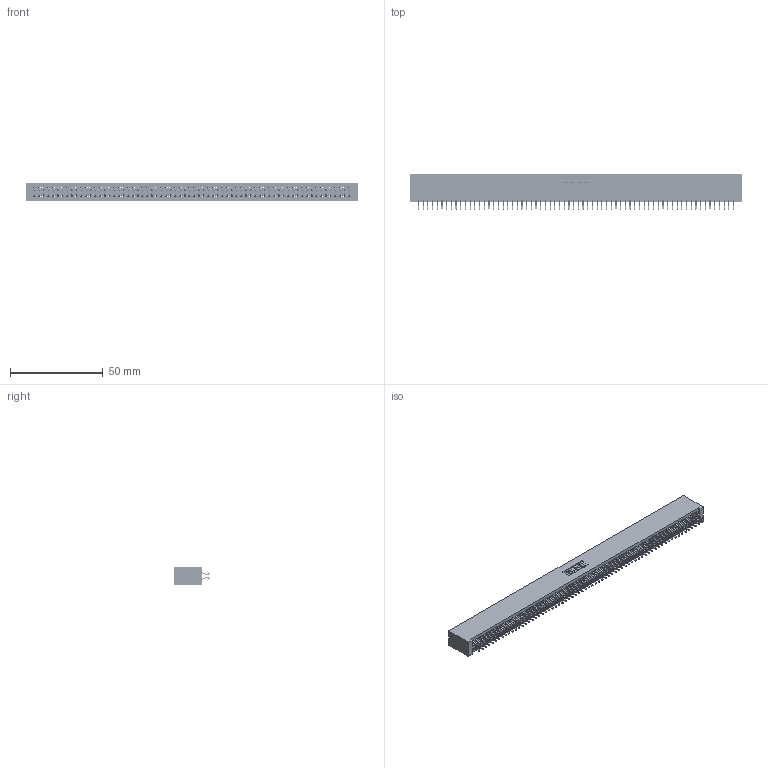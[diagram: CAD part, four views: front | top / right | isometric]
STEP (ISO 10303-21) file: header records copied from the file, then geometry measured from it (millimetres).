
FILE_DESCRIPTION (( 'STEP AP203' ), '1' );
FILE_NAME ('395-136-556-201.STEP', '2018-12-05T10:28:58', ( '' ), ( '' ), 'SwSTEP 2.0', 'SolidWorks 2016', '' );
FILE_SCHEMA (( 'CONFIG_CONTROL_DESIGN' ));
Length unit declared in the file: inch
Products named in the file (3): 395-136-556-201; 345-292-001_556 Tail; 345 Part_No Mounting Lugs
Assembly tree (137 placements, depth 2):
  395-136-556-201
    345 Part_No Mounting Lugs
    345-292-001_556 Tail  x136
Bounding box: 179.32 x 19.24 x 9.4 mm (x, y, z)
Volume: 18271.6 mm3; surface area: 27696.3 mm2
Topology: 137 solids, 137 shells, 7734 faces, 23029 edges, 15170 vertices
Faces by surface type: plane 5108, cylinder 2626
Entity records: 49797 total; most frequent: CARTESIAN_POINT 8336, ORIENTED_EDGE 8258, DIRECTION 7301, EDGE_CURVE 4129, LINE 3725, VECTOR 3725, VERTEX_POINT 2750, AXIS2_PLACEMENT_3D 1788
